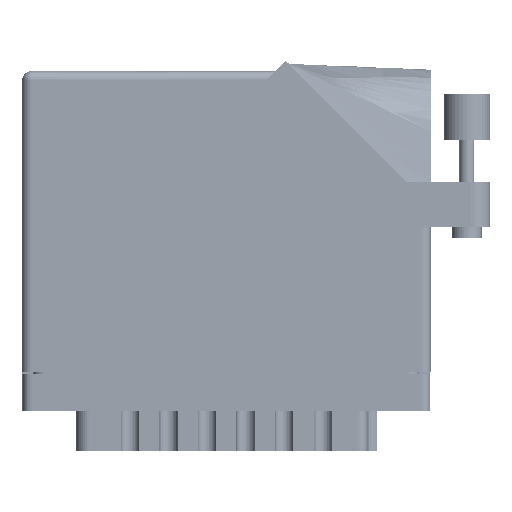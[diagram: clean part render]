
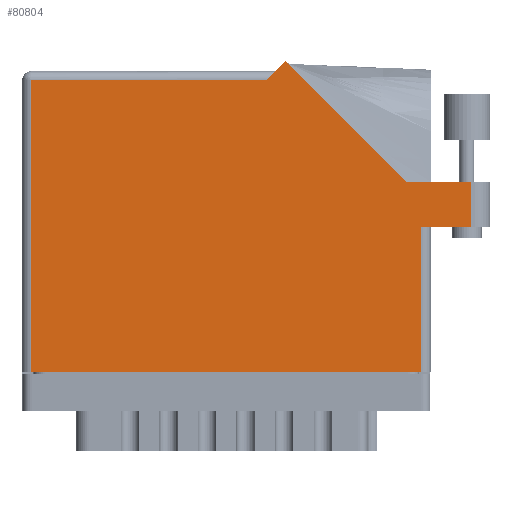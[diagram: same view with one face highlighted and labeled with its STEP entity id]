
A CAD part, front view. The second image highlights one B-rep face of the part: STEP entity #80804.
In plain terms, the highlighted face is planar.
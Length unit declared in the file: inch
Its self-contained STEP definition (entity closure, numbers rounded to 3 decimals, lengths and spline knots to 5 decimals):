
#263 = ORIENTED_EDGE ( 'NONE', *, *, #59743, .T. ) ;
#535 = VERTEX_POINT ( 'NONE', #27872 ) ;
#1279 = EDGE_CURVE ( 'NONE', #59953, #535, #84708, .T. ) ;
#2591 = ORIENTED_EDGE ( 'NONE', *, *, #1279, .T. ) ;
#3301 = FACE_OUTER_BOUND ( 'NONE', #30289, .T. ) ;
#3891 = ORIENTED_EDGE ( 'NONE', *, *, #42214, .T. ) ;
#4428 = ORIENTED_EDGE ( 'NONE', *, *, #9557, .T. ) ;
#4692 = CARTESIAN_POINT ( 'NONE',  ( 3.03, 0.98, 0. ) ) ;
#5898 = ORIENTED_EDGE ( 'NONE', *, *, #8112, .T. ) ;
#8112 = EDGE_CURVE ( 'NONE', #64068, #36851, #68544, .T. ) ;
#9557 = EDGE_CURVE ( 'NONE', #36241, #50450, #33357, .T. ) ;
#10658 = VERTEX_POINT ( 'NONE', #36936 ) ;
#10860 = EDGE_CURVE ( 'NONE', #83234, #64068, #60873, .T. ) ;
#12142 = VECTOR ( 'NONE', #76236, 39.37008 ) ;
#13234 = CARTESIAN_POINT ( 'NONE',  ( 0.062, 1.968, 0. ) ) ;
#14781 = CARTESIAN_POINT ( 'NONE',  ( 0., 2.03, 0. ) ) ;
#16721 = CARTESIAN_POINT ( 'NONE',  ( 0., 1.968, 0. ) ) ;
#18131 = EDGE_CURVE ( 'NONE', #10658, #83234, #84096, .T. ) ;
#18567 = VECTOR ( 'NONE', #58019, 39.37008 ) ;
#18781 = LINE ( 'NONE', #63401, #26652 ) ;
#19590 = DIRECTION ( 'NONE',  ( -0.707, -0.707, 0. ) ) ;
#22334 = LINE ( 'NONE', #69016, #12142 ) ;
#23473 = VECTOR ( 'NONE', #51798, 39.37008 ) ;
#24841 = VERTEX_POINT ( 'NONE', #91412 ) ;
#26652 = VECTOR ( 'NONE', #19590, 39.37008 ) ;
#27872 = CARTESIAN_POINT ( 'NONE',  ( 2.693, 0., 0. ) ) ;
#28547 = CARTESIAN_POINT ( 'NONE',  ( 0.062, 0., 0. ) ) ;
#29649 = LINE ( 'NONE', #59530, #59858 ) ;
#30289 = EDGE_LOOP ( 'NONE', ( #50378, #61818, #5898, #263, #84338, #4428, #3891, #2591, #35598 ) ) ;
#31663 = CARTESIAN_POINT ( 'NONE',  ( 1.643, 1.968, 0. ) ) ;
#33357 = LINE ( 'NONE', #16721, #72479 ) ;
#34000 = CARTESIAN_POINT ( 'NONE',  ( 0.062, 0., 0. ) ) ;
#35598 = ORIENTED_EDGE ( 'NONE', *, *, #82705, .T. ) ;
#35905 = AXIS2_PLACEMENT_3D ( 'NONE', #14781, #78112, #86587 ) ;
#36241 = VERTEX_POINT ( 'NONE', #31663 ) ;
#36851 = VERTEX_POINT ( 'NONE', #60898 ) ;
#36936 = CARTESIAN_POINT ( 'NONE',  ( 2.693, 0.98, 0. ) ) ;
#38088 = DIRECTION ( 'NONE',  ( -1., 0., 0. ) ) ;
#42214 = EDGE_CURVE ( 'NONE', #50450, #59953, #59797, .T. ) ;
#42693 = PLANE ( 'NONE',  #35905 ) ;
#47466 = VECTOR ( 'NONE', #76003, 39.37008 ) ;
#47583 = VECTOR ( 'NONE', #84161, 39.37008 ) ;
#49540 = VECTOR ( 'NONE', #75510, 39.37008 ) ;
#50378 = ORIENTED_EDGE ( 'NONE', *, *, #18131, .T. ) ;
#50450 = VERTEX_POINT ( 'NONE', #13234 ) ;
#51798 = DIRECTION ( 'NONE',  ( 1., 0., 0. ) ) ;
#55229 = CARTESIAN_POINT ( 'NONE',  ( 3.03, 1.287, 0. ) ) ;
#58019 = DIRECTION ( 'NONE',  ( 1., 0., 0. ) ) ;
#59530 = CARTESIAN_POINT ( 'NONE',  ( 2.58942, 1.287, 0. ) ) ;
#59743 = EDGE_CURVE ( 'NONE', #36851, #24841, #29649, .T. ) ;
#59797 = LINE ( 'NONE', #34000, #47583 ) ;
#59858 = VECTOR ( 'NONE', #66161, 39.37008 ) ;
#59953 = VERTEX_POINT ( 'NONE', #28547 ) ;
#60873 = LINE ( 'NONE', #68476, #47466 ) ;
#60898 = CARTESIAN_POINT ( 'NONE',  ( 2.58942, 1.287, 0. ) ) ;
#61066 = EDGE_CURVE ( 'NONE', #24841, #36241, #18781, .T. ) ;
#61818 = ORIENTED_EDGE ( 'NONE', *, *, #10860, .T. ) ;
#63401 = CARTESIAN_POINT ( 'NONE',  ( 1.705, 2.03, 0. ) ) ;
#64068 = VERTEX_POINT ( 'NONE', #55229 ) ;
#65866 = CARTESIAN_POINT ( 'NONE',  ( 0., 0., 0. ) ) ;
#66161 = DIRECTION ( 'NONE',  ( -0.707, 0.707, 0. ) ) ;
#68476 = CARTESIAN_POINT ( 'NONE',  ( 3.03, 1.287, 0. ) ) ;
#68544 = LINE ( 'NONE', #83704, #49540 ) ;
#69016 = CARTESIAN_POINT ( 'NONE',  ( 2.693, 0.98, 0. ) ) ;
#72479 = VECTOR ( 'NONE', #38088, 39.37008 ) ;
#75510 = DIRECTION ( 'NONE',  ( -1., 0., 0. ) ) ;
#76003 = DIRECTION ( 'NONE',  ( 0., 1., 0. ) ) ;
#76236 = DIRECTION ( 'NONE',  ( 0., 1., 0. ) ) ;
#78112 = DIRECTION ( 'NONE',  ( 0., 0., -1. ) ) ;
#79384 = CARTESIAN_POINT ( 'NONE',  ( 2.755, 0.98, 0. ) ) ;
#80804 = ADVANCED_FACE ( 'NONE', ( #3301 ), #42693, .F. ) ;
#82705 = EDGE_CURVE ( 'NONE', #535, #10658, #22334, .T. ) ;
#83234 = VERTEX_POINT ( 'NONE', #4692 ) ;
#83704 = CARTESIAN_POINT ( 'NONE',  ( 3.155, 1.287, 0. ) ) ;
#84096 = LINE ( 'NONE', #79384, #23473 ) ;
#84161 = DIRECTION ( 'NONE',  ( 0., -1., 0. ) ) ;
#84338 = ORIENTED_EDGE ( 'NONE', *, *, #61066, .T. ) ;
#84708 = LINE ( 'NONE', #65866, #18567 ) ;
#86587 = DIRECTION ( 'NONE',  ( -1., 0., 0. ) ) ;
#91412 = CARTESIAN_POINT ( 'NONE',  ( 1.77571, 2.10071, 0. ) ) ;
